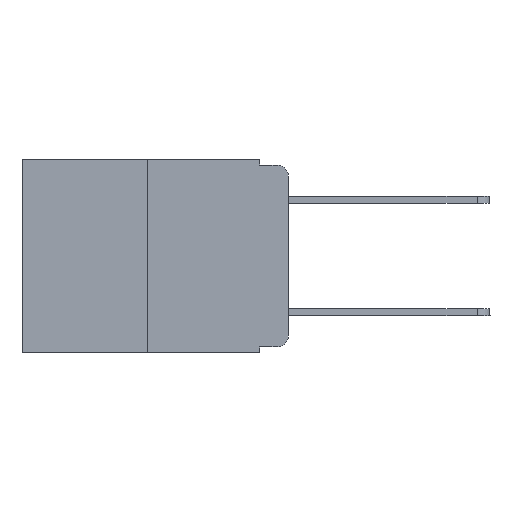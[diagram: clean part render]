
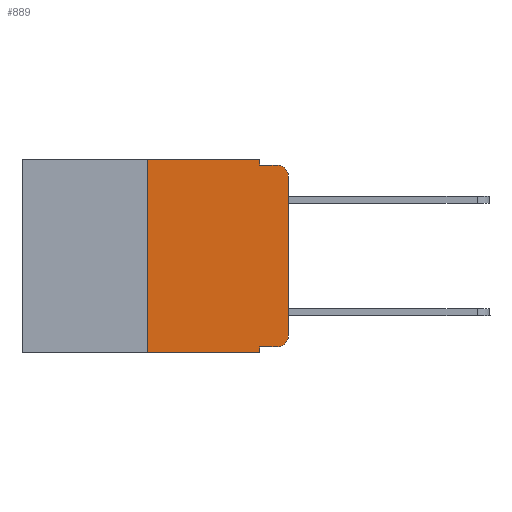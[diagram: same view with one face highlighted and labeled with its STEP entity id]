
A CAD part, left-side view. The second image highlights one B-rep face of the part: STEP entity #889.
In plain terms, the highlighted planar face has unit normal (-1, 0, 0).
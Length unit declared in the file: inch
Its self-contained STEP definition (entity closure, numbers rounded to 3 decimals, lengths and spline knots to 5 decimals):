
#70 = CARTESIAN_POINT ( 'NONE',  ( 0., 0.02, -0.313 ) ) ;
#116 = DIRECTION ( 'NONE',  ( 0., -1., 0. ) ) ;
#207 = EDGE_CURVE ( 'NONE', #7495, #15707, #8576, .T. ) ;
#634 = EDGE_LOOP ( 'NONE', ( #18104, #11280, #6920, #21182, #1841, #10846, #15989, #9178, #2163, #9060 ) ) ;
#662 = VECTOR ( 'NONE', #6075, 39.37008 ) ;
#864 = LINE ( 'NONE', #20391, #16110 ) ;
#889 = ADVANCED_FACE ( 'NONE', ( #20087 ), #7580, .F. ) ;
#1297 = EDGE_CURVE ( 'NONE', #6386, #6481, #11221, .T. ) ;
#1375 = AXIS2_PLACEMENT_3D ( 'NONE', #3765, #12940, #20206 ) ;
#1579 = DIRECTION ( 'NONE',  ( 0., 0., -1. ) ) ;
#1677 = CARTESIAN_POINT ( 'NONE',  ( 0., 0., 0. ) ) ;
#1841 = ORIENTED_EDGE ( 'NONE', *, *, #10329, .F. ) ;
#2163 = ORIENTED_EDGE ( 'NONE', *, *, #17927, .T. ) ;
#2288 = DIRECTION ( 'NONE',  ( 0., -1., 0. ) ) ;
#2605 = EDGE_CURVE ( 'NONE', #4110, #14228, #16243, .T. ) ;
#2884 = CARTESIAN_POINT ( 'NONE',  ( 0., 0.02, -0.333 ) ) ;
#3148 = VECTOR ( 'NONE', #8927, 39.37008 ) ;
#3327 = EDGE_CURVE ( 'NONE', #4110, #11295, #864, .T. ) ;
#3473 = CARTESIAN_POINT ( 'NONE',  ( 0., 0.051, 0. ) ) ;
#3634 = DIRECTION ( 'NONE',  ( -1., 0., 0. ) ) ;
#3675 = CARTESIAN_POINT ( 'NONE',  ( 0., 0.051, -0.01 ) ) ;
#3765 = CARTESIAN_POINT ( 'NONE',  ( 0., 0.473, 0. ) ) ;
#3984 = DIRECTION ( 'NONE',  ( 0., -1., 0. ) ) ;
#4110 = VERTEX_POINT ( 'NONE', #5664 ) ;
#4242 = CARTESIAN_POINT ( 'NONE',  ( 0., 0., -0.03 ) ) ;
#5664 = CARTESIAN_POINT ( 'NONE',  ( 0., 0.25, -0.343 ) ) ;
#5721 = CARTESIAN_POINT ( 'NONE',  ( 0., 0.051, 0. ) ) ;
#5760 = EDGE_CURVE ( 'NONE', #16786, #7495, #18132, .T. ) ;
#6075 = DIRECTION ( 'NONE',  ( 0., 0., -1. ) ) ;
#6386 = VERTEX_POINT ( 'NONE', #17842 ) ;
#6449 = VERTEX_POINT ( 'NONE', #7482 ) ;
#6481 = VERTEX_POINT ( 'NONE', #16644 ) ;
#6920 = ORIENTED_EDGE ( 'NONE', *, *, #22691, .F. ) ;
#7482 = CARTESIAN_POINT ( 'NONE',  ( 0., 0.02, -0.01 ) ) ;
#7495 = VERTEX_POINT ( 'NONE', #18870 ) ;
#7580 = PLANE ( 'NONE',  #1375 ) ;
#7712 = VECTOR ( 'NONE', #3984, 39.37008 ) ;
#7870 = AXIS2_PLACEMENT_3D ( 'NONE', #70, #3634, #14241 ) ;
#8576 = LINE ( 'NONE', #1677, #3148 ) ;
#8927 = DIRECTION ( 'NONE',  ( 0., 0., 1. ) ) ;
#9060 = ORIENTED_EDGE ( 'NONE', *, *, #5760, .T. ) ;
#9086 = CARTESIAN_POINT ( 'NONE',  ( 0., 0.051, -0.343 ) ) ;
#9178 = ORIENTED_EDGE ( 'NONE', *, *, #12671, .F. ) ;
#10329 = EDGE_CURVE ( 'NONE', #11295, #6386, #23300, .T. ) ;
#10846 = ORIENTED_EDGE ( 'NONE', *, *, #3327, .F. ) ;
#11221 = LINE ( 'NONE', #5721, #662 ) ;
#11280 = ORIENTED_EDGE ( 'NONE', *, *, #18338, .T. ) ;
#11295 = VERTEX_POINT ( 'NONE', #18114 ) ;
#11336 = LINE ( 'NONE', #13236, #11889 ) ;
#11889 = VECTOR ( 'NONE', #2288, 39.37008 ) ;
#12671 = EDGE_CURVE ( 'NONE', #23458, #14228, #17885, .T. ) ;
#12940 = DIRECTION ( 'NONE',  ( 1., 0., 0. ) ) ;
#13035 = CARTESIAN_POINT ( 'NONE',  ( 0., 0.473, -0.343 ) ) ;
#13236 = CARTESIAN_POINT ( 'NONE',  ( 0., 0.051, -0.333 ) ) ;
#14228 = VERTEX_POINT ( 'NONE', #9086 ) ;
#14241 = DIRECTION ( 'NONE',  ( 0., 0., -1. ) ) ;
#14389 = LINE ( 'NONE', #3675, #15763 ) ;
#14646 = CARTESIAN_POINT ( 'NONE',  ( 0., 0.02, -0.03 ) ) ;
#14850 = VECTOR ( 'NONE', #23071, 39.37008 ) ;
#14950 = CIRCLE ( 'NONE', #20284, 0.02 ) ;
#15536 = CARTESIAN_POINT ( 'NONE',  ( 0., 0.051, -0.333 ) ) ;
#15707 = VERTEX_POINT ( 'NONE', #4242 ) ;
#15763 = VECTOR ( 'NONE', #116, 39.37008 ) ;
#15989 = ORIENTED_EDGE ( 'NONE', *, *, #2605, .T. ) ;
#16110 = VECTOR ( 'NONE', #20754, 39.37008 ) ;
#16243 = LINE ( 'NONE', #13035, #7712 ) ;
#16644 = CARTESIAN_POINT ( 'NONE',  ( 0., 0.051, -0.01 ) ) ;
#16786 = VERTEX_POINT ( 'NONE', #2884 ) ;
#17511 = VECTOR ( 'NONE', #1579, 39.37008 ) ;
#17563 = CARTESIAN_POINT ( 'NONE',  ( 0., 0.473, 0. ) ) ;
#17842 = CARTESIAN_POINT ( 'NONE',  ( 0., 0.051, 0. ) ) ;
#17885 = LINE ( 'NONE', #3473, #17511 ) ;
#17927 = EDGE_CURVE ( 'NONE', #23458, #16786, #11336, .T. ) ;
#18104 = ORIENTED_EDGE ( 'NONE', *, *, #207, .T. ) ;
#18114 = CARTESIAN_POINT ( 'NONE',  ( 0., 0.25, 0. ) ) ;
#18132 = CIRCLE ( 'NONE', #7870, 0.02 ) ;
#18338 = EDGE_CURVE ( 'NONE', #15707, #6449, #14950, .T. ) ;
#18691 = DIRECTION ( 'NONE',  ( 0., 0., -1. ) ) ;
#18870 = CARTESIAN_POINT ( 'NONE',  ( 0., 0., -0.313 ) ) ;
#20087 = FACE_OUTER_BOUND ( 'NONE', #634, .T. ) ;
#20206 = DIRECTION ( 'NONE',  ( 0., 0., -1. ) ) ;
#20254 = DIRECTION ( 'NONE',  ( -1., 0., 0. ) ) ;
#20284 = AXIS2_PLACEMENT_3D ( 'NONE', #14646, #20254, #18691 ) ;
#20391 = CARTESIAN_POINT ( 'NONE',  ( 0., 0.25, 0. ) ) ;
#20754 = DIRECTION ( 'NONE',  ( 0., 0., 1. ) ) ;
#21182 = ORIENTED_EDGE ( 'NONE', *, *, #1297, .F. ) ;
#22691 = EDGE_CURVE ( 'NONE', #6481, #6449, #14389, .T. ) ;
#23071 = DIRECTION ( 'NONE',  ( 0., -1., 0. ) ) ;
#23300 = LINE ( 'NONE', #17563, #14850 ) ;
#23458 = VERTEX_POINT ( 'NONE', #15536 ) ;
